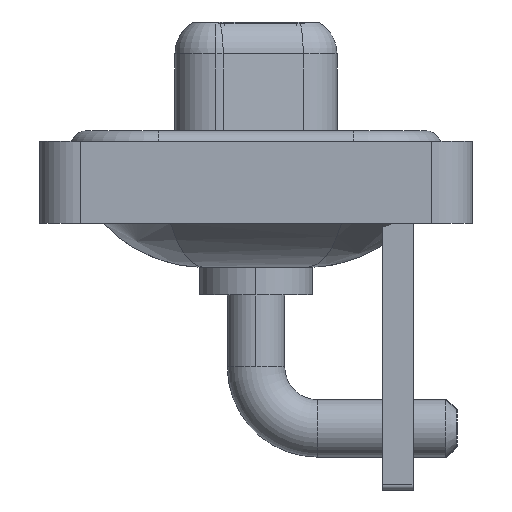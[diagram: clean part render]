
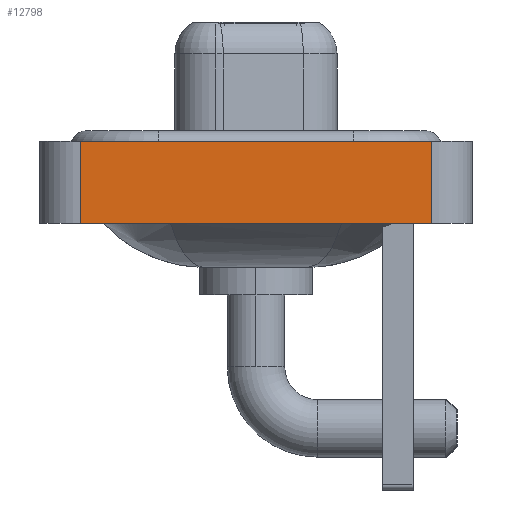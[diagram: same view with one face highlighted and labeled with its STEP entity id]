
A CAD part, left-side view. The second image highlights one B-rep face of the part: STEP entity #12798.
In plain terms, the highlighted planar face has unit normal (-1, 0, 0).
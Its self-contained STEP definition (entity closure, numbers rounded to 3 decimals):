
#46 = VERTEX_POINT ( 'NONE', #15549 ) ;
#1047 = CARTESIAN_POINT ( 'NONE',  ( -7.3, -8.55, -3.6 ) ) ;
#1518 = CARTESIAN_POINT ( 'NONE',  ( -7.3, 8.55, -3.6 ) ) ;
#1744 = DIRECTION ( 'NONE',  ( 0., 0., 1. ) ) ;
#1862 = LINE ( 'NONE', #10323, #10855 ) ;
#2380 = CARTESIAN_POINT ( 'NONE',  ( -7.3, -8.55, -3.6 ) ) ;
#3309 = CARTESIAN_POINT ( 'NONE',  ( -7.3, 8.55, -3.6 ) ) ;
#3424 = VERTEX_POINT ( 'NONE', #1518 ) ;
#5229 = FACE_OUTER_BOUND ( 'NONE', #18106, .T. ) ;
#5468 = VECTOR ( 'NONE', #12241, 1000. ) ;
#6705 = DIRECTION ( 'NONE',  ( -1., 0., 0. ) ) ;
#6927 = CARTESIAN_POINT ( 'NONE',  ( -7.3, -8.55, 0.4 ) ) ;
#6952 = CARTESIAN_POINT ( 'NONE',  ( -7.3, -8.55, -3.6 ) ) ;
#7036 = EDGE_CURVE ( 'NONE', #46, #11043, #9990, .T. ) ;
#7539 = DIRECTION ( 'NONE',  ( 0., 0., 1. ) ) ;
#7640 = ORIENTED_EDGE ( 'NONE', *, *, #12627, .T. ) ;
#8461 = VERTEX_POINT ( 'NONE', #2380 ) ;
#8889 = LINE ( 'NONE', #3309, #12342 ) ;
#8926 = ORIENTED_EDGE ( 'NONE', *, *, #13896, .F. ) ;
#9990 = LINE ( 'NONE', #6927, #16738 ) ;
#10323 = CARTESIAN_POINT ( 'NONE',  ( -7.3, -8.55, -3.6 ) ) ;
#10855 = VECTOR ( 'NONE', #7539, 1000. ) ;
#10890 = CARTESIAN_POINT ( 'NONE',  ( -7.3, -8.55, 0.4 ) ) ;
#11043 = VERTEX_POINT ( 'NONE', #10890 ) ;
#11311 = EDGE_CURVE ( 'NONE', #3424, #8461, #16709, .T. ) ;
#12241 = DIRECTION ( 'NONE',  ( 0., -1., 0. ) ) ;
#12342 = VECTOR ( 'NONE', #1744, 1000. ) ;
#12627 = EDGE_CURVE ( 'NONE', #8461, #11043, #1862, .T. ) ;
#12798 = ADVANCED_FACE ( 'NONE', ( #5229 ), #16561, .T. ) ;
#13896 = EDGE_CURVE ( 'NONE', #3424, #46, #8889, .T. ) ;
#14947 = ORIENTED_EDGE ( 'NONE', *, *, #7036, .F. ) ;
#15549 = CARTESIAN_POINT ( 'NONE',  ( -7.3, 8.55, 0.4 ) ) ;
#15675 = DIRECTION ( 'NONE',  ( 0., -1., 0. ) ) ;
#16508 = AXIS2_PLACEMENT_3D ( 'NONE', #1047, #6705, #18030 ) ;
#16561 = PLANE ( 'NONE',  #16508 ) ;
#16709 = LINE ( 'NONE', #6952, #5468 ) ;
#16738 = VECTOR ( 'NONE', #15675, 1000. ) ;
#17487 = ORIENTED_EDGE ( 'NONE', *, *, #11311, .T. ) ;
#18030 = DIRECTION ( 'NONE',  ( 0., 0., 1. ) ) ;
#18106 = EDGE_LOOP ( 'NONE', ( #7640, #14947, #8926, #17487 ) ) ;
